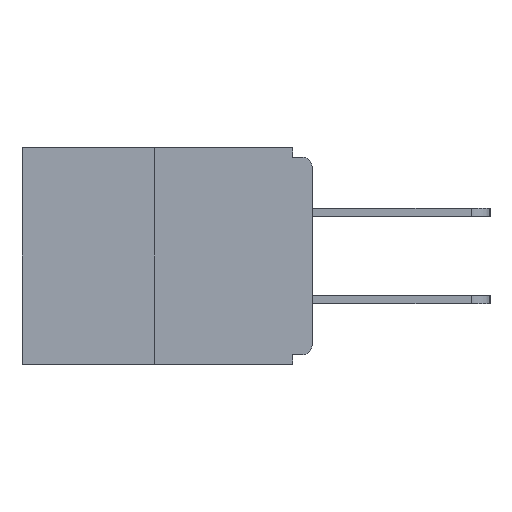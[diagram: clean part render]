
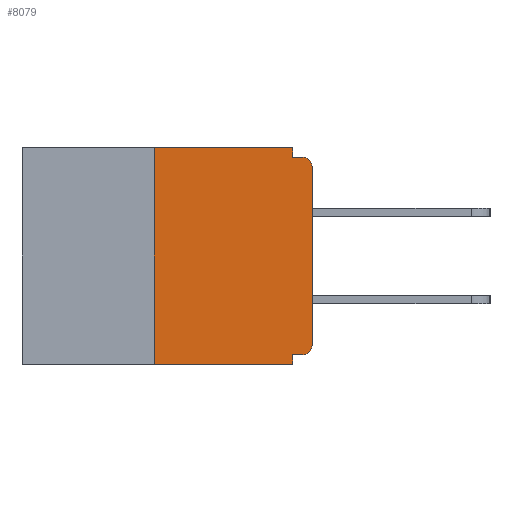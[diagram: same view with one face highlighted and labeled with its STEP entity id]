
A CAD part, left-side view. The second image highlights one B-rep face of the part: STEP entity #8079.
In plain terms, the highlighted planar face has unit normal (-1, 0, 0).
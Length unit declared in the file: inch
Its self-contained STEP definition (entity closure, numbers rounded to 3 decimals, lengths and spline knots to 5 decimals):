
#10 = DIRECTION ( 'NONE',  ( 0., 0., -1. ) ) ;
#163 = DIRECTION ( 'NONE',  ( 0., -1., 0. ) ) ;
#227 = CIRCLE ( 'NONE', #4594, 0.015 ) ;
#250 = EDGE_CURVE ( 'NONE', #12042, #4885, #8963, .T. ) ;
#691 = VECTOR ( 'NONE', #9899, 39.37008 ) ;
#795 = EDGE_CURVE ( 'NONE', #6054, #5784, #10018, .T. ) ;
#799 = CARTESIAN_POINT ( 'NONE',  ( 0., 0.031, -0.015 ) ) ;
#878 = AXIS2_PLACEMENT_3D ( 'NONE', #5286, #4290, #9077 ) ;
#898 = ORIENTED_EDGE ( 'NONE', *, *, #2971, .T. ) ;
#942 = DIRECTION ( 'NONE',  ( 0., 0., -1. ) ) ;
#988 = ORIENTED_EDGE ( 'NONE', *, *, #4807, .F. ) ;
#1095 = LINE ( 'NONE', #4858, #10944 ) ;
#1455 = DIRECTION ( 'NONE',  ( 1., 0., 0. ) ) ;
#1656 = CIRCLE ( 'NONE', #878, 0.015 ) ;
#1716 = VECTOR ( 'NONE', #10, 39.37008 ) ;
#1835 = EDGE_CURVE ( 'NONE', #4037, #7812, #227, .T. ) ;
#1997 = DIRECTION ( 'NONE',  ( 0., 0., 1. ) ) ;
#2600 = EDGE_LOOP ( 'NONE', ( #5978, #3558, #6768, #8398, #9093, #898, #6375, #10409, #988, #2895 ) ) ;
#2662 = LINE ( 'NONE', #8571, #1716 ) ;
#2671 = CARTESIAN_POINT ( 'NONE',  ( 0., 0.46, 0. ) ) ;
#2709 = VERTEX_POINT ( 'NONE', #6626 ) ;
#2858 = EDGE_CURVE ( 'NONE', #6322, #4037, #5805, .T. ) ;
#2882 = EDGE_CURVE ( 'NONE', #4885, #2709, #9585, .T. ) ;
#2895 = ORIENTED_EDGE ( 'NONE', *, *, #8601, .F. ) ;
#2971 = EDGE_CURVE ( 'NONE', #12042, #6322, #1656, .T. ) ;
#3232 = CARTESIAN_POINT ( 'NONE',  ( 0., 0.031, -0.328 ) ) ;
#3238 = DIRECTION ( 'NONE',  ( 0., 1., 0. ) ) ;
#3558 = ORIENTED_EDGE ( 'NONE', *, *, #8810, .F. ) ;
#3917 = DIRECTION ( 'NONE',  ( 0., 0., -1. ) ) ;
#4037 = VERTEX_POINT ( 'NONE', #11933 ) ;
#4187 = CARTESIAN_POINT ( 'NONE',  ( 0., 0.25, -0.343 ) ) ;
#4290 = DIRECTION ( 'NONE',  ( -1., 0., 0. ) ) ;
#4485 = PLANE ( 'NONE',  #8875 ) ;
#4594 = AXIS2_PLACEMENT_3D ( 'NONE', #5645, #9442, #942 ) ;
#4796 = CARTESIAN_POINT ( 'NONE',  ( 0., 0., 0. ) ) ;
#4807 = EDGE_CURVE ( 'NONE', #9259, #7812, #1095, .T. ) ;
#4858 = CARTESIAN_POINT ( 'NONE',  ( 0., 0., -0.015 ) ) ;
#4878 = DIRECTION ( 'NONE',  ( 0., -1., 0. ) ) ;
#4885 = VERTEX_POINT ( 'NONE', #3232 ) ;
#5118 = VERTEX_POINT ( 'NONE', #4187 ) ;
#5281 = CARTESIAN_POINT ( 'NONE',  ( 0., 0.46, 0. ) ) ;
#5286 = CARTESIAN_POINT ( 'NONE',  ( 0., 0.015, -0.313 ) ) ;
#5303 = EDGE_CURVE ( 'NONE', #5118, #2709, #9674, .T. ) ;
#5355 = CARTESIAN_POINT ( 'NONE',  ( 0., 0.25, 0. ) ) ;
#5422 = FACE_OUTER_BOUND ( 'NONE', #2600, .T. ) ;
#5645 = CARTESIAN_POINT ( 'NONE',  ( 0., 0.015, -0.03 ) ) ;
#5687 = VECTOR ( 'NONE', #10187, 39.37008 ) ;
#5784 = VERTEX_POINT ( 'NONE', #9530 ) ;
#5805 = LINE ( 'NONE', #4796, #5836 ) ;
#5836 = VECTOR ( 'NONE', #1997, 39.37008 ) ;
#5861 = CARTESIAN_POINT ( 'NONE',  ( 0., 0., -0.313 ) ) ;
#5978 = ORIENTED_EDGE ( 'NONE', *, *, #795, .F. ) ;
#6054 = VERTEX_POINT ( 'NONE', #5355 ) ;
#6322 = VERTEX_POINT ( 'NONE', #5861 ) ;
#6375 = ORIENTED_EDGE ( 'NONE', *, *, #2858, .T. ) ;
#6626 = CARTESIAN_POINT ( 'NONE',  ( 0., 0.031, -0.343 ) ) ;
#6666 = VECTOR ( 'NONE', #3238, 39.37008 ) ;
#6697 = CARTESIAN_POINT ( 'NONE',  ( 0., 0.015, -0.015 ) ) ;
#6768 = ORIENTED_EDGE ( 'NONE', *, *, #5303, .T. ) ;
#7279 = CARTESIAN_POINT ( 'NONE',  ( 0., 0.25, 0. ) ) ;
#7812 = VERTEX_POINT ( 'NONE', #6697 ) ;
#7978 = CARTESIAN_POINT ( 'NONE',  ( 0., 0., -0.328 ) ) ;
#8079 = ADVANCED_FACE ( 'NONE', ( #5422 ), #4485, .F. ) ;
#8290 = DIRECTION ( 'NONE',  ( 0., 0., -1. ) ) ;
#8398 = ORIENTED_EDGE ( 'NONE', *, *, #2882, .F. ) ;
#8571 = CARTESIAN_POINT ( 'NONE',  ( 0., 0.031, 0. ) ) ;
#8601 = EDGE_CURVE ( 'NONE', #5784, #9259, #2662, .T. ) ;
#8645 = CARTESIAN_POINT ( 'NONE',  ( 0., 0.031, -0.343 ) ) ;
#8810 = EDGE_CURVE ( 'NONE', #5118, #6054, #8999, .T. ) ;
#8875 = AXIS2_PLACEMENT_3D ( 'NONE', #2671, #1455, #8290 ) ;
#8963 = LINE ( 'NONE', #7978, #6666 ) ;
#8999 = LINE ( 'NONE', #7279, #5687 ) ;
#9077 = DIRECTION ( 'NONE',  ( 0., 0., -1. ) ) ;
#9093 = ORIENTED_EDGE ( 'NONE', *, *, #250, .F. ) ;
#9259 = VERTEX_POINT ( 'NONE', #799 ) ;
#9305 = CARTESIAN_POINT ( 'NONE',  ( 0., 0.015, -0.328 ) ) ;
#9442 = DIRECTION ( 'NONE',  ( -1., 0., 0. ) ) ;
#9530 = CARTESIAN_POINT ( 'NONE',  ( 0., 0.031, 0. ) ) ;
#9585 = LINE ( 'NONE', #8645, #9787 ) ;
#9674 = LINE ( 'NONE', #12247, #11972 ) ;
#9787 = VECTOR ( 'NONE', #3917, 39.37008 ) ;
#9899 = DIRECTION ( 'NONE',  ( 0., -1., 0. ) ) ;
#10018 = LINE ( 'NONE', #5281, #691 ) ;
#10187 = DIRECTION ( 'NONE',  ( 0., 0., 1. ) ) ;
#10409 = ORIENTED_EDGE ( 'NONE', *, *, #1835, .T. ) ;
#10944 = VECTOR ( 'NONE', #163, 39.37008 ) ;
#11933 = CARTESIAN_POINT ( 'NONE',  ( 0., 0., -0.03 ) ) ;
#11972 = VECTOR ( 'NONE', #4878, 39.37008 ) ;
#12042 = VERTEX_POINT ( 'NONE', #9305 ) ;
#12247 = CARTESIAN_POINT ( 'NONE',  ( 0., 0.46, -0.343 ) ) ;
